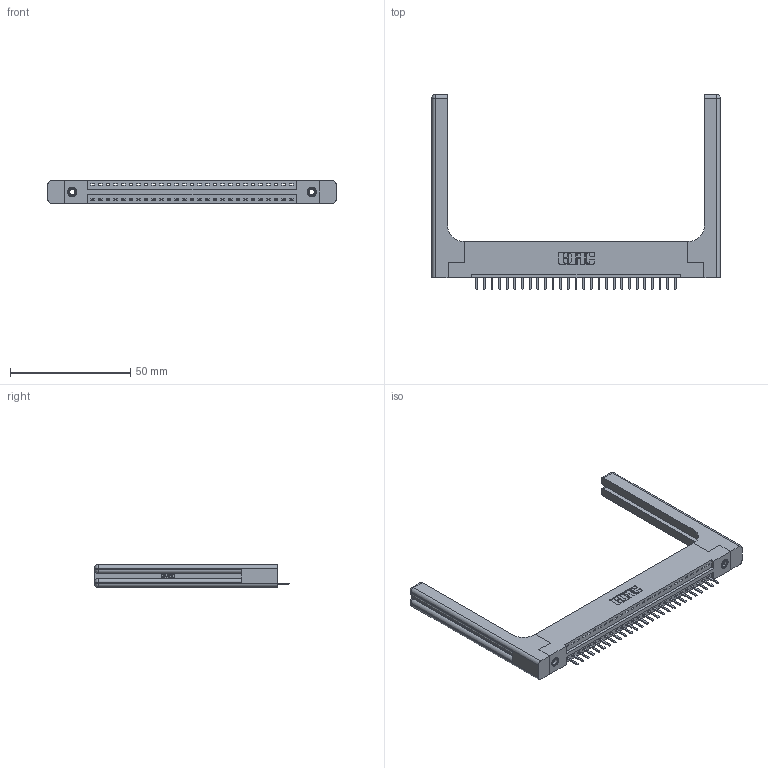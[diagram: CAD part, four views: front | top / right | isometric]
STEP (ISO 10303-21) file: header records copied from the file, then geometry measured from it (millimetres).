
FILE_DESCRIPTION (( 'STEP AP203' ), '1' );
FILE_NAME ('396-027-520-158.STEP', '2019-10-27T07:38:19', ( '' ), ( '' ), 'SwSTEP 2.0', 'SolidWorks 2016', '' );
FILE_SCHEMA (( 'CONFIG_CONTROL_DESIGN' ));
Length unit declared in the file: inch
Products named in the file (5): 345-250-001_345-250-001-102; 345-292-001_345-293-120; 396-027-520-158; 346-220-058_345-220-058; 346 Part_Flush Mounting Lugs - 0.156 Dia-TH
Assembly tree (32 placements, depth 2):
  396-027-520-158
    346 Part_Flush Mounting Lugs - 0.156 Dia-TH
    345-292-001_345-293-120  x27
    345-250-001_345-250-001-102  x2
    346-220-058_345-220-058  x2
Bounding box: 119.79 x 80.98 x 9.4 mm (x, y, z)
Volume: 18803.6 mm3; surface area: 18853.4 mm2
Topology: 32 solids, 32 shells, 2052 faces, 5963 edges, 3882 vertices
Faces by surface type: plane 1358, cylinder 634, bspline 36, cone 12, sphere 8, torus 4
Entity records: 24072 total; most frequent: CARTESIAN_POINT 5122, ORIENTED_EDGE 3868, DIRECTION 3456, EDGE_CURVE 1934, VECTOR 1598, LINE 1598, VERTEX_POINT 1278, AXIS2_PLACEMENT_3D 929
